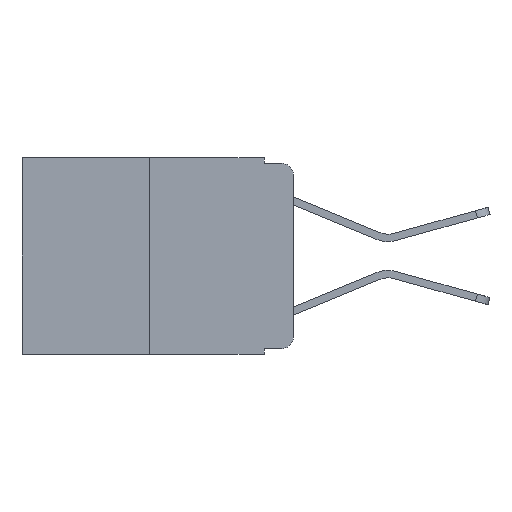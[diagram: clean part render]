
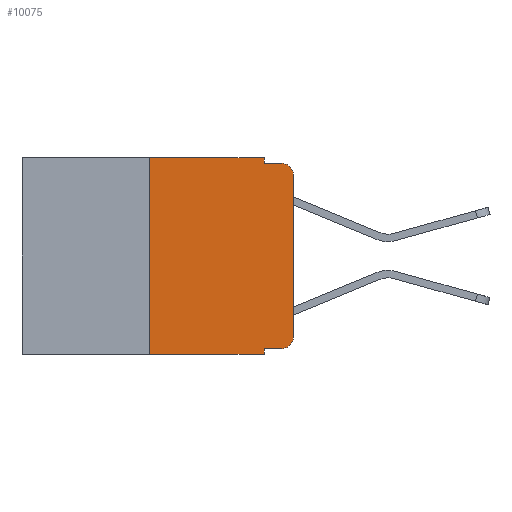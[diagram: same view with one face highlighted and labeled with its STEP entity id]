
A CAD part, left-side view. The second image highlights one B-rep face of the part: STEP entity #10075.
In plain terms, the highlighted planar face has unit normal (-1, 0, 0).
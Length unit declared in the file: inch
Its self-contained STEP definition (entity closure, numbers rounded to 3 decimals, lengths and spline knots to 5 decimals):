
#65 = LINE ( 'NONE', #3166, #8321 ) ;
#117 = CARTESIAN_POINT ( 'NONE',  ( 0., 0.051, 0. ) ) ;
#122 = CARTESIAN_POINT ( 'NONE',  ( 0., 0.051, -0.01 ) ) ;
#320 = PLANE ( 'NONE',  #12059 ) ;
#392 = CARTESIAN_POINT ( 'NONE',  ( 0., 0.051, -0.343 ) ) ;
#549 = EDGE_CURVE ( 'NONE', #5428, #1714, #966, .T. ) ;
#595 = CIRCLE ( 'NONE', #10741, 0.02 ) ;
#910 = VECTOR ( 'NONE', #5453, 39.37008 ) ;
#951 = ORIENTED_EDGE ( 'NONE', *, *, #10715, .F. ) ;
#966 = LINE ( 'NONE', #9216, #10340 ) ;
#989 = CARTESIAN_POINT ( 'NONE',  ( 0., 0., -0.313 ) ) ;
#1383 = LINE ( 'NONE', #10778, #910 ) ;
#1536 = EDGE_CURVE ( 'NONE', #12771, #8933, #1383, .T. ) ;
#1714 = VERTEX_POINT ( 'NONE', #8011 ) ;
#2049 = EDGE_LOOP ( 'NONE', ( #3866, #10807, #3022, #2842, #12680, #10179, #7144, #951, #4807, #2406 ) ) ;
#2406 = ORIENTED_EDGE ( 'NONE', *, *, #7146, .T. ) ;
#2842 = ORIENTED_EDGE ( 'NONE', *, *, #12857, .F. ) ;
#2867 = VERTEX_POINT ( 'NONE', #117 ) ;
#3022 = ORIENTED_EDGE ( 'NONE', *, *, #549, .F. ) ;
#3096 = CARTESIAN_POINT ( 'NONE',  ( 0., 0.051, -0.333 ) ) ;
#3166 = CARTESIAN_POINT ( 'NONE',  ( 0., 0., 0. ) ) ;
#3537 = DIRECTION ( 'NONE',  ( 0., 0., -1. ) ) ;
#3656 = DIRECTION ( 'NONE',  ( 0., 0., -1. ) ) ;
#3676 = AXIS2_PLACEMENT_3D ( 'NONE', #4563, #11657, #3537 ) ;
#3727 = CARTESIAN_POINT ( 'NONE',  ( 0., 0.051, 0. ) ) ;
#3866 = ORIENTED_EDGE ( 'NONE', *, *, #13180, .T. ) ;
#4158 = VERTEX_POINT ( 'NONE', #392 ) ;
#4302 = VECTOR ( 'NONE', #9711, 39.37008 ) ;
#4345 = CARTESIAN_POINT ( 'NONE',  ( 0., 0.25, 0. ) ) ;
#4563 = CARTESIAN_POINT ( 'NONE',  ( 0., 0.02, -0.313 ) ) ;
#4619 = VERTEX_POINT ( 'NONE', #8692 ) ;
#4807 = ORIENTED_EDGE ( 'NONE', *, *, #12622, .T. ) ;
#5049 = DIRECTION ( 'NONE',  ( 0., 0., -1. ) ) ;
#5317 = VERTEX_POINT ( 'NONE', #3096 ) ;
#5428 = VERTEX_POINT ( 'NONE', #122 ) ;
#5430 = CARTESIAN_POINT ( 'NONE',  ( 0., 0.25, -0.343 ) ) ;
#5453 = DIRECTION ( 'NONE',  ( 0., 0., 1. ) ) ;
#5539 = EDGE_CURVE ( 'NONE', #12771, #4158, #10734, .T. ) ;
#5672 = EDGE_CURVE ( 'NONE', #4619, #1714, #595, .T. ) ;
#6501 = CIRCLE ( 'NONE', #3676, 0.02 ) ;
#6623 = DIRECTION ( 'NONE',  ( 1., 0., 0. ) ) ;
#6960 = DIRECTION ( 'NONE',  ( -1., 0., 0. ) ) ;
#7144 = ORIENTED_EDGE ( 'NONE', *, *, #5539, .T. ) ;
#7146 = EDGE_CURVE ( 'NONE', #9297, #10497, #6501, .T. ) ;
#7896 = VECTOR ( 'NONE', #3656, 39.37008 ) ;
#8011 = CARTESIAN_POINT ( 'NONE',  ( 0., 0.02, -0.01 ) ) ;
#8321 = VECTOR ( 'NONE', #9268, 39.37008 ) ;
#8692 = CARTESIAN_POINT ( 'NONE',  ( 0., 0., -0.03 ) ) ;
#8694 = CARTESIAN_POINT ( 'NONE',  ( 0., 0.051, 0. ) ) ;
#8833 = LINE ( 'NONE', #8694, #4302 ) ;
#8933 = VERTEX_POINT ( 'NONE', #4345 ) ;
#9216 = CARTESIAN_POINT ( 'NONE',  ( 0., 0.051, -0.01 ) ) ;
#9268 = DIRECTION ( 'NONE',  ( 0., 0., 1. ) ) ;
#9285 = DIRECTION ( 'NONE',  ( 0., -1., 0. ) ) ;
#9297 = VERTEX_POINT ( 'NONE', #10677 ) ;
#9458 = FACE_OUTER_BOUND ( 'NONE', #2049, .T. ) ;
#9499 = LINE ( 'NONE', #10641, #10321 ) ;
#9611 = VECTOR ( 'NONE', #9285, 39.37008 ) ;
#9658 = DIRECTION ( 'NONE',  ( 0., 0., -1. ) ) ;
#9711 = DIRECTION ( 'NONE',  ( 0., 0., -1. ) ) ;
#9885 = VECTOR ( 'NONE', #11742, 39.37008 ) ;
#9945 = LINE ( 'NONE', #3727, #7896 ) ;
#10075 = ADVANCED_FACE ( 'NONE', ( #9458 ), #320, .F. ) ;
#10179 = ORIENTED_EDGE ( 'NONE', *, *, #1536, .F. ) ;
#10287 = CARTESIAN_POINT ( 'NONE',  ( 0., 0.051, -0.333 ) ) ;
#10321 = VECTOR ( 'NONE', #10373, 39.37008 ) ;
#10340 = VECTOR ( 'NONE', #12261, 39.37008 ) ;
#10373 = DIRECTION ( 'NONE',  ( 0., -1., 0. ) ) ;
#10497 = VERTEX_POINT ( 'NONE', #989 ) ;
#10641 = CARTESIAN_POINT ( 'NONE',  ( 0., 0.473, 0. ) ) ;
#10677 = CARTESIAN_POINT ( 'NONE',  ( 0., 0.02, -0.333 ) ) ;
#10715 = EDGE_CURVE ( 'NONE', #5317, #4158, #8833, .T. ) ;
#10734 = LINE ( 'NONE', #12780, #9885 ) ;
#10741 = AXIS2_PLACEMENT_3D ( 'NONE', #12978, #6960, #5049 ) ;
#10778 = CARTESIAN_POINT ( 'NONE',  ( 0., 0.25, 0. ) ) ;
#10807 = ORIENTED_EDGE ( 'NONE', *, *, #5672, .T. ) ;
#10967 = EDGE_CURVE ( 'NONE', #8933, #2867, #9499, .T. ) ;
#11657 = DIRECTION ( 'NONE',  ( -1., 0., 0. ) ) ;
#11681 = CARTESIAN_POINT ( 'NONE',  ( 0., 0.473, 0. ) ) ;
#11742 = DIRECTION ( 'NONE',  ( 0., -1., 0. ) ) ;
#12059 = AXIS2_PLACEMENT_3D ( 'NONE', #11681, #6623, #9658 ) ;
#12261 = DIRECTION ( 'NONE',  ( 0., -1., 0. ) ) ;
#12326 = LINE ( 'NONE', #10287, #9611 ) ;
#12622 = EDGE_CURVE ( 'NONE', #5317, #9297, #12326, .T. ) ;
#12680 = ORIENTED_EDGE ( 'NONE', *, *, #10967, .F. ) ;
#12771 = VERTEX_POINT ( 'NONE', #5430 ) ;
#12780 = CARTESIAN_POINT ( 'NONE',  ( 0., 0.473, -0.343 ) ) ;
#12857 = EDGE_CURVE ( 'NONE', #2867, #5428, #9945, .T. ) ;
#12978 = CARTESIAN_POINT ( 'NONE',  ( 0., 0.02, -0.03 ) ) ;
#13180 = EDGE_CURVE ( 'NONE', #10497, #4619, #65, .T. ) ;
